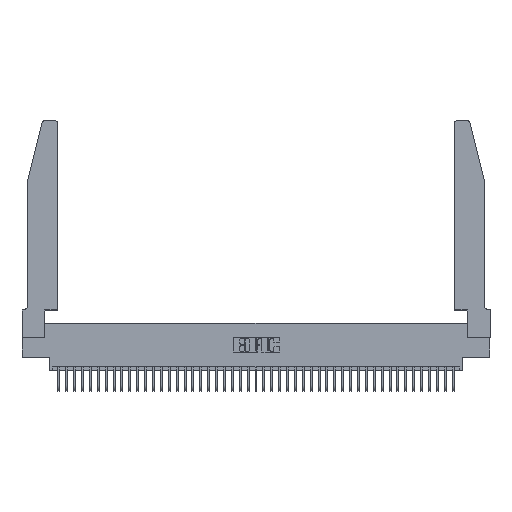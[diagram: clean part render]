
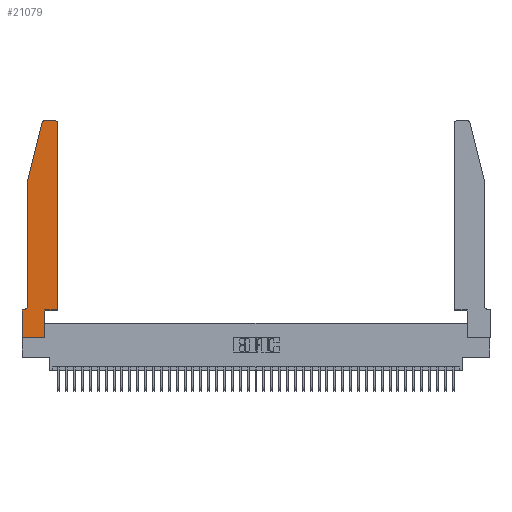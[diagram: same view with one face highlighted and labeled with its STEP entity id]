
A CAD part, top view. The second image highlights one B-rep face of the part: STEP entity #21079.
In plain terms, the highlighted planar face has unit normal (0, 0, 1).
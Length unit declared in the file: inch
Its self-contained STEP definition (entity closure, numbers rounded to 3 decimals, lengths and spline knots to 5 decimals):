
#24 = AXIS2_PLACEMENT_3D ( 'NONE', #8030, #30867, #11291 ) ;
#379 = EDGE_CURVE ( 'NONE', #4393, #37473, #37444, .T. ) ;
#831 = ORIENTED_EDGE ( 'NONE', *, *, #34445, .T. ) ;
#1526 = LINE ( 'NONE', #30626, #16805 ) ;
#2356 = DIRECTION ( 'NONE',  ( 1., 0., 0. ) ) ;
#2526 = ORIENTED_EDGE ( 'NONE', *, *, #12371, .T. ) ;
#3516 = ORIENTED_EDGE ( 'NONE', *, *, #379, .T. ) ;
#3584 = PLANE ( 'NONE',  #16600 ) ;
#4393 = VERTEX_POINT ( 'NONE', #32135 ) ;
#4839 = LINE ( 'NONE', #39143, #21148 ) ;
#6180 = ORIENTED_EDGE ( 'NONE', *, *, #15084, .T. ) ;
#6498 = EDGE_CURVE ( 'NONE', #7456, #19061, #4839, .T. ) ;
#6714 = CARTESIAN_POINT ( 'NONE',  ( 0., 0.35, 0.37 ) ) ;
#6723 = LINE ( 'NONE', #15543, #15405 ) ;
#6856 = DIRECTION ( 'NONE',  ( 0., 0., 1. ) ) ;
#7456 = VERTEX_POINT ( 'NONE', #21363 ) ;
#8030 = CARTESIAN_POINT ( 'NONE',  ( 0.4205, 2.72, 0.37 ) ) ;
#8571 = CARTESIAN_POINT ( 'NONE',  ( 0.0055, 0.42, 0.37 ) ) ;
#8993 = CARTESIAN_POINT ( 'NONE',  ( 0.0755, 2., 0.37 ) ) ;
#9226 = ORIENTED_EDGE ( 'NONE', *, *, #15075, .T. ) ;
#9478 = AXIS2_PLACEMENT_3D ( 'NONE', #36094, #16645, #39343 ) ;
#10490 = FACE_OUTER_BOUND ( 'NONE', #35669, .T. ) ;
#10798 = ORIENTED_EDGE ( 'NONE', *, *, #6498, .T. ) ;
#11187 = CARTESIAN_POINT ( 'NONE',  ( 0., 0., 0.37 ) ) ;
#11291 = DIRECTION ( 'NONE',  ( 1., 0., 0. ) ) ;
#11835 = DIRECTION ( 'NONE',  ( -1., 0., 0. ) ) ;
#12095 = LINE ( 'NONE', #11187, #13144 ) ;
#12371 = EDGE_CURVE ( 'NONE', #25678, #7456, #20947, .T. ) ;
#12389 = DIRECTION ( 'NONE',  ( 0., 1., 0. ) ) ;
#13144 = VECTOR ( 'NONE', #33852, 39.37008 ) ;
#13583 = LINE ( 'NONE', #14023, #29921 ) ;
#13758 = EDGE_CURVE ( 'NONE', #25019, #39908, #25434, .T. ) ;
#14023 = CARTESIAN_POINT ( 'NONE',  ( 0.2605, 2.75, 0.37 ) ) ;
#14968 = CARTESIAN_POINT ( 'NONE',  ( 0.2865, 0., 0.37 ) ) ;
#15075 = EDGE_CURVE ( 'NONE', #41338, #25678, #23838, .T. ) ;
#15084 = EDGE_CURVE ( 'NONE', #39908, #40259, #15185, .T. ) ;
#15185 = LINE ( 'NONE', #35153, #22831 ) ;
#15405 = VECTOR ( 'NONE', #38216, 39.37008 ) ;
#15543 = CARTESIAN_POINT ( 'NONE',  ( 0.4505, 0.35, 0.37 ) ) ;
#15682 = DIRECTION ( 'NONE',  ( 0., -1., 0. ) ) ;
#16445 = DIRECTION ( 'NONE',  ( -1., 0., 0. ) ) ;
#16600 = AXIS2_PLACEMENT_3D ( 'NONE', #6714, #6856, #29670 ) ;
#16645 = DIRECTION ( 'NONE',  ( 0., 0., 1. ) ) ;
#16711 = EDGE_CURVE ( 'NONE', #40259, #20851, #27672, .T. ) ;
#16748 = VECTOR ( 'NONE', #2356, 39.37008 ) ;
#16805 = VECTOR ( 'NONE', #33988, 39.37008 ) ;
#17651 = CARTESIAN_POINT ( 'NONE',  ( 0., 0.35, 0.37 ) ) ;
#18661 = CARTESIAN_POINT ( 'NONE',  ( 0.4505, 0.35, 0.37 ) ) ;
#18978 = VECTOR ( 'NONE', #40531, 39.37008 ) ;
#19061 = VERTEX_POINT ( 'NONE', #17651 ) ;
#19771 = EDGE_CURVE ( 'NONE', #19061, #25019, #12095, .T. ) ;
#20720 = VERTEX_POINT ( 'NONE', #34350 ) ;
#20851 = VERTEX_POINT ( 'NONE', #18661 ) ;
#20947 = CIRCLE ( 'NONE', #24771, 0.07 ) ;
#21079 = ADVANCED_FACE ( 'NONE', ( #10490 ), #3584, .T. ) ;
#21116 = CARTESIAN_POINT ( 'NONE',  ( 0.4505, 0.35, 0.37 ) ) ;
#21148 = VECTOR ( 'NONE', #16445, 39.37008 ) ;
#21363 = CARTESIAN_POINT ( 'NONE',  ( 0.0055, 0.35, 0.37 ) ) ;
#22491 = EDGE_CURVE ( 'NONE', #25252, #4393, #13583, .T. ) ;
#22831 = VECTOR ( 'NONE', #12389, 39.37008 ) ;
#23838 = LINE ( 'NONE', #31937, #24856 ) ;
#24771 = AXIS2_PLACEMENT_3D ( 'NONE', #8571, #31398, #11835 ) ;
#24856 = VECTOR ( 'NONE', #15682, 39.37008 ) ;
#25019 = VERTEX_POINT ( 'NONE', #36279 ) ;
#25252 = VERTEX_POINT ( 'NONE', #28532 ) ;
#25434 = LINE ( 'NONE', #31563, #16748 ) ;
#25678 = VERTEX_POINT ( 'NONE', #35744 ) ;
#26166 = CARTESIAN_POINT ( 'NONE',  ( 0.25487, 2.72718, 0.37 ) ) ;
#26743 = CARTESIAN_POINT ( 'NONE',  ( 0.2865, 0.35, 0.37 ) ) ;
#27672 = LINE ( 'NONE', #21116, #18978 ) ;
#28041 = ORIENTED_EDGE ( 'NONE', *, *, #30925, .T. ) ;
#28532 = CARTESIAN_POINT ( 'NONE',  ( 0.4205, 2.75, 0.37 ) ) ;
#29360 = ORIENTED_EDGE ( 'NONE', *, *, #16711, .T. ) ;
#29670 = DIRECTION ( 'NONE',  ( 1., 0., 0. ) ) ;
#29921 = VECTOR ( 'NONE', #36585, 39.37008 ) ;
#30626 = CARTESIAN_POINT ( 'NONE',  ( 0.0755, 2., 0.37 ) ) ;
#30867 = DIRECTION ( 'NONE',  ( 0., 0., 1. ) ) ;
#30925 = EDGE_CURVE ( 'NONE', #20851, #20720, #6723, .T. ) ;
#31398 = DIRECTION ( 'NONE',  ( 0., 0., -1. ) ) ;
#31563 = CARTESIAN_POINT ( 'NONE',  ( 0., 0., 0.37 ) ) ;
#31937 = CARTESIAN_POINT ( 'NONE',  ( 0.0755, 2., 0.37 ) ) ;
#32135 = CARTESIAN_POINT ( 'NONE',  ( 0.284, 2.75, 0.37 ) ) ;
#32673 = ORIENTED_EDGE ( 'NONE', *, *, #37736, .T. ) ;
#33852 = DIRECTION ( 'NONE',  ( 0., -1., 0. ) ) ;
#33988 = DIRECTION ( 'NONE',  ( -0.239, -0.971, 0. ) ) ;
#34350 = CARTESIAN_POINT ( 'NONE',  ( 0.4505, 2.72, 0.37 ) ) ;
#34445 = EDGE_CURVE ( 'NONE', #37473, #41338, #1526, .T. ) ;
#35153 = CARTESIAN_POINT ( 'NONE',  ( 0.2865, 0.35, 0.37 ) ) ;
#35669 = EDGE_LOOP ( 'NONE', ( #39563, #3516, #831, #9226, #2526, #10798, #39624, #36789, #6180, #29360, #28041, #32673 ) ) ;
#35744 = CARTESIAN_POINT ( 'NONE',  ( 0.0755, 0.42, 0.37 ) ) ;
#36094 = CARTESIAN_POINT ( 'NONE',  ( 0.284, 2.72, 0.37 ) ) ;
#36279 = CARTESIAN_POINT ( 'NONE',  ( 0., 0., 0.37 ) ) ;
#36585 = DIRECTION ( 'NONE',  ( -1., 0., 0. ) ) ;
#36789 = ORIENTED_EDGE ( 'NONE', *, *, #13758, .T. ) ;
#37330 = CIRCLE ( 'NONE', #24, 0.03 ) ;
#37444 = CIRCLE ( 'NONE', #9478, 0.03 ) ;
#37473 = VERTEX_POINT ( 'NONE', #26166 ) ;
#37736 = EDGE_CURVE ( 'NONE', #20720, #25252, #37330, .T. ) ;
#38216 = DIRECTION ( 'NONE',  ( 0., 1., 0. ) ) ;
#39143 = CARTESIAN_POINT ( 'NONE',  ( 0.0755, 0.35, 0.37 ) ) ;
#39343 = DIRECTION ( 'NONE',  ( 1., 0., 0. ) ) ;
#39563 = ORIENTED_EDGE ( 'NONE', *, *, #22491, .T. ) ;
#39624 = ORIENTED_EDGE ( 'NONE', *, *, #19771, .T. ) ;
#39908 = VERTEX_POINT ( 'NONE', #14968 ) ;
#40259 = VERTEX_POINT ( 'NONE', #26743 ) ;
#40531 = DIRECTION ( 'NONE',  ( 1., 0., 0. ) ) ;
#41338 = VERTEX_POINT ( 'NONE', #8993 ) ;
